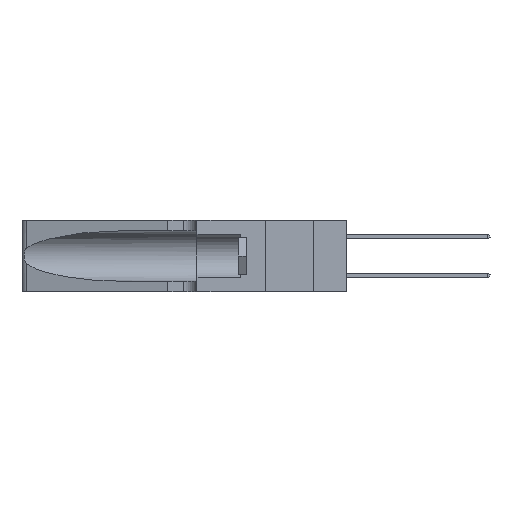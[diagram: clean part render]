
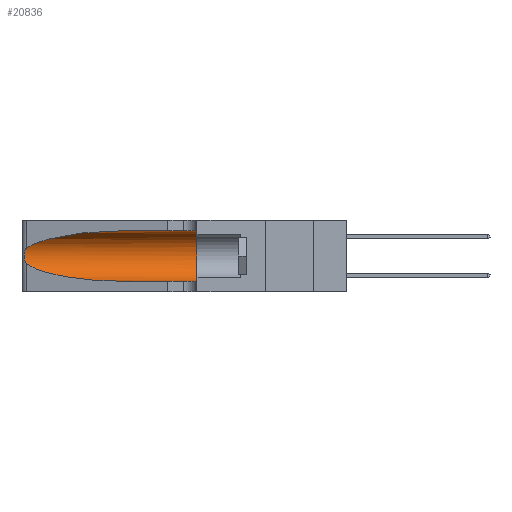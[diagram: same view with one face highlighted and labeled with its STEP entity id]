
A CAD part, left-side view. The second image highlights one B-rep face of the part: STEP entity #20836.
In plain terms, the highlighted cylindrical face has radius 3.308 mm (diameter 6.617 mm), a partial arc.
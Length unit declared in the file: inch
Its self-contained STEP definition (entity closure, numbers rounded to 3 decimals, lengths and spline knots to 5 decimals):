
#718 = CARTESIAN_POINT ( 'NONE',  ( 0.25487, 1.22718, 0.22369 ) ) ;
#920 = FACE_OUTER_BOUND ( 'NONE', #15549, .T. ) ;
#1629 = DIRECTION ( 'NONE',  ( 0., 1., 0. ) ) ;
#2936 = DIRECTION ( 'NONE',  ( 0., -1., 0. ) ) ;
#2984 = CARTESIAN_POINT ( 'NONE',  ( 0.25487, 1.22718, 0.14631 ) ) ;
#3388 = CARTESIAN_POINT ( 'NONE',  ( 0.25787, 1.23484, 0.2124 ) ) ;
#3511 = CARTESIAN_POINT ( 'NONE',  ( 0.25487, 1.22718, 0.14631 ) ) ;
#3903 = ORIENTED_EDGE ( 'NONE', *, *, #29437, .T. ) ;
#4277 = EDGE_CURVE ( 'NONE', #8617, #10813, #10630, .T. ) ;
#4469 = CARTESIAN_POINT ( 'NONE',  ( 0.1305, 1.61858, 0.31525 ) ) ;
#5563 = CARTESIAN_POINT ( 'NONE',  ( 0.2373, 1.15595, 0.08982 ) ) ;
#5944 = CARTESIAN_POINT ( 'NONE',  ( 0.26018, 1.23835, 0.19895 ) ) ;
#7037 = DIRECTION ( 'NONE',  ( 0., -1., 0. ) ) ;
#7049 = EDGE_CURVE ( 'NONE', #30604, #28845, #29751, .T. ) ;
#8504 = CARTESIAN_POINT ( 'NONE',  ( 0.26075, 1.23896, 0.178 ) ) ;
#8617 = VERTEX_POINT ( 'NONE', #14331 ) ;
#9784 =( BOUNDED_CURVE ( )  B_SPLINE_CURVE ( 3, ( #2984, #5563, #28253, #13220 ),
 .UNSPECIFIED., .F., .T. ) 
 B_SPLINE_CURVE_WITH_KNOTS ( ( 4, 4 ),
 ( 3.44316, 4.71239 ),
 .UNSPECIFIED. ) 
 CURVE ( )  GEOMETRIC_REPRESENTATION_ITEM ( )  RATIONAL_B_SPLINE_CURVE ( ( 1., 0.87, 0.87, 1. ) ) 
 REPRESENTATION_ITEM ( '' )  );
#9825 = VECTOR ( 'NONE', #22655, 39.37008 ) ;
#9834 = CARTESIAN_POINT ( 'NONE',  ( 0.25487, 1.22718, 0.22369 ) ) ;
#10031 = CARTESIAN_POINT ( 'NONE',  ( 0.1305, 0.35, 0.31525 ) ) ;
#10515 = DIRECTION ( 'NONE',  ( 0., 0., -1. ) ) ;
#10630 = LINE ( 'NONE', #32622, #9825 ) ;
#10813 = VERTEX_POINT ( 'NONE', #27582 ) ;
#10974 = CARTESIAN_POINT ( 'NONE',  ( 0.25639, 1.23184, 0.21858 ) ) ;
#11068 = ORIENTED_EDGE ( 'NONE', *, *, #24541, .F. ) ;
#11089 = CARTESIAN_POINT ( 'NONE',  ( 0.25856, 1.23593, 0.16098 ) ) ;
#12245 =( BOUNDED_CURVE ( )  B_SPLINE_CURVE ( 3, ( #28439, #30944, #15944, #718 ),
 .UNSPECIFIED., .F., .F. ) 
 B_SPLINE_CURVE_WITH_KNOTS ( ( 4, 4 ),
 ( 1.5708, 2.84003 ),
 .UNSPECIFIED. ) 
 CURVE ( )  GEOMETRIC_REPRESENTATION_ITEM ( )  RATIONAL_B_SPLINE_CURVE ( ( 1., 0.87, 0.87, 1. ) ) 
 REPRESENTATION_ITEM ( '' )  );
#12760 = VERTEX_POINT ( 'NONE', #27803 ) ;
#13220 = CARTESIAN_POINT ( 'NONE',  ( 0.1305, 0.72297, 0.05475 ) ) ;
#13324 = VECTOR ( 'NONE', #7037, 39.37008 ) ;
#13623 = CARTESIAN_POINT ( 'NONE',  ( 0.25639, 1.23186, 0.15144 ) ) ;
#13667 = CYLINDRICAL_SURFACE ( 'NONE', #31257, 0.13025 ) ;
#14258 = EDGE_CURVE ( 'NONE', #12760, #30604, #12245, .T. ) ;
#14331 = CARTESIAN_POINT ( 'NONE',  ( 0.1305, 0.72297, 0.05475 ) ) ;
#15549 = EDGE_LOOP ( 'NONE', ( #20211, #25010, #3903, #24177, #11068, #29458 ) ) ;
#15944 = CARTESIAN_POINT ( 'NONE',  ( 0.2373, 1.15595, 0.28018 ) ) ;
#16154 = CARTESIAN_POINT ( 'NONE',  ( 0.25487, 1.22718, 0.14631 ) ) ;
#16849 = CARTESIAN_POINT ( 'NONE',  ( 0.1305, 0.35, 0.185 ) ) ;
#17748 = VERTEX_POINT ( 'NONE', #10031 ) ;
#18565 = CARTESIAN_POINT ( 'NONE',  ( 0.25487, 1.22718, 0.22369 ) ) ;
#19347 = DIRECTION ( 'NONE',  ( 0., 0., 1. ) ) ;
#20211 = ORIENTED_EDGE ( 'NONE', *, *, #14258, .T. ) ;
#20836 = ADVANCED_FACE ( 'NONE', ( #920 ), #13667, .F. ) ;
#21058 = CARTESIAN_POINT ( 'NONE',  ( 0.25854, 1.2359, 0.20912 ) ) ;
#22655 = DIRECTION ( 'NONE',  ( 0., -1., 0. ) ) ;
#22728 = AXIS2_PLACEMENT_3D ( 'NONE', #16849, #1629, #19347 ) ;
#23584 = CARTESIAN_POINT ( 'NONE',  ( 0.26075, 1.23896, 0.19203 ) ) ;
#24177 = ORIENTED_EDGE ( 'NONE', *, *, #4277, .T. ) ;
#24541 = EDGE_CURVE ( 'NONE', #17748, #10813, #28384, .T. ) ;
#25010 = ORIENTED_EDGE ( 'NONE', *, *, #7049, .T. ) ;
#26124 = CARTESIAN_POINT ( 'NONE',  ( 0.26017, 1.23833, 0.17102 ) ) ;
#26675 = LINE ( 'NONE', #4469, #13324 ) ;
#27124 = EDGE_CURVE ( 'NONE', #12760, #17748, #26675, .T. ) ;
#27582 = CARTESIAN_POINT ( 'NONE',  ( 0.1305, 0.35, 0.05475 ) ) ;
#27803 = CARTESIAN_POINT ( 'NONE',  ( 0.1305, 0.72297, 0.31525 ) ) ;
#28253 = CARTESIAN_POINT ( 'NONE',  ( 0.18966, 0.96281, 0.05475 ) ) ;
#28384 = CIRCLE ( 'NONE', #22728, 0.13025 ) ;
#28439 = CARTESIAN_POINT ( 'NONE',  ( 0.1305, 0.72297, 0.31525 ) ) ;
#28546 = CARTESIAN_POINT ( 'NONE',  ( 0.25555, 1.22994, 0.2215 ) ) ;
#28648 = CARTESIAN_POINT ( 'NONE',  ( 0.25789, 1.23486, 0.15765 ) ) ;
#28845 = VERTEX_POINT ( 'NONE', #3511 ) ;
#29437 = EDGE_CURVE ( 'NONE', #28845, #8617, #9784, .T. ) ;
#29458 = ORIENTED_EDGE ( 'NONE', *, *, #27124, .F. ) ;
#29751 = B_SPLINE_CURVE_WITH_KNOTS ( 'NONE', 3,
 ( #18565, #28546, #10974, #3388, #21058, #5944, #23584, #8504, #26124, #11089, #28648, #13623, #31162, #16154 ),
 .UNSPECIFIED., .F., .F.,
 ( 4, 2, 2, 2, 2, 2, 4 ),
 ( 0., 0.00027, 0.00053, 0.00107, 0.0016, 0.00187, 0.00214 ),
 .UNSPECIFIED. ) ;
#30604 = VERTEX_POINT ( 'NONE', #9834 ) ;
#30622 = CARTESIAN_POINT ( 'NONE',  ( 0.1305, 1.61858, 0.185 ) ) ;
#30944 = CARTESIAN_POINT ( 'NONE',  ( 0.18966, 0.96281, 0.31525 ) ) ;
#31162 = CARTESIAN_POINT ( 'NONE',  ( 0.25555, 1.22993, 0.14849 ) ) ;
#31257 = AXIS2_PLACEMENT_3D ( 'NONE', #30622, #2936, #10515 ) ;
#32622 = CARTESIAN_POINT ( 'NONE',  ( 0.1305, 1.61858, 0.05475 ) ) ;
